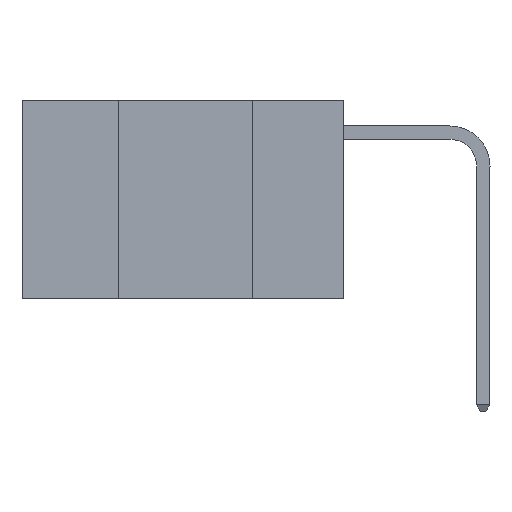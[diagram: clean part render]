
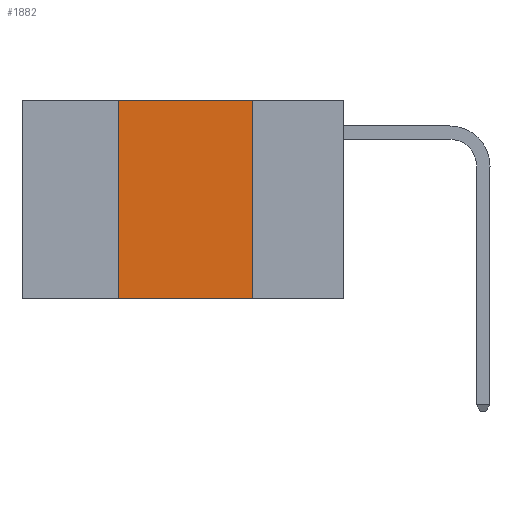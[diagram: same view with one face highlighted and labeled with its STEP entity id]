
A CAD part, left-side view. The second image highlights one B-rep face of the part: STEP entity #1882.
In plain terms, the highlighted planar face has unit normal (-1, 0, 0).
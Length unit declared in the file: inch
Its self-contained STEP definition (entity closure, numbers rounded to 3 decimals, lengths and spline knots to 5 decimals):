
#71 = EDGE_CURVE ( 'NONE', #2229, #2671, #3245, .T. ) ;
#581 = EDGE_CURVE ( 'NONE', #2229, #3153, #977, .T. ) ;
#640 = EDGE_LOOP ( 'NONE', ( #3433, #2370, #1067, #1055 ) ) ;
#672 = CARTESIAN_POINT ( 'NONE',  ( 0., 0.42, 0. ) ) ;
#694 = FACE_OUTER_BOUND ( 'NONE', #640, .T. ) ;
#722 = VECTOR ( 'NONE', #8742, 39.37008 ) ;
#977 = LINE ( 'NONE', #672, #722 ) ;
#986 = VECTOR ( 'NONE', #7277, 39.37008 ) ;
#1055 = ORIENTED_EDGE ( 'NONE', *, *, #71, .T. ) ;
#1067 = ORIENTED_EDGE ( 'NONE', *, *, #581, .F. ) ;
#1360 = AXIS2_PLACEMENT_3D ( 'NONE', #4078, #2463, #3861 ) ;
#1510 = CARTESIAN_POINT ( 'NONE',  ( 0., 0.42, 0. ) ) ;
#1602 = VERTEX_POINT ( 'NONE', #4942 ) ;
#1882 = ADVANCED_FACE ( 'NONE', ( #694 ), #4094, .F. ) ;
#2224 = DIRECTION ( 'NONE',  ( 0., 0., -1. ) ) ;
#2229 = VERTEX_POINT ( 'NONE', #7825 ) ;
#2370 = ORIENTED_EDGE ( 'NONE', *, *, #3351, .F. ) ;
#2463 = DIRECTION ( 'NONE',  ( 1., 0., 0. ) ) ;
#2671 = VERTEX_POINT ( 'NONE', #3814 ) ;
#3137 = EDGE_CURVE ( 'NONE', #1602, #2671, #6580, .T. ) ;
#3153 = VERTEX_POINT ( 'NONE', #1510 ) ;
#3245 = LINE ( 'NONE', #5629, #986 ) ;
#3351 = EDGE_CURVE ( 'NONE', #3153, #1602, #5281, .T. ) ;
#3433 = ORIENTED_EDGE ( 'NONE', *, *, #3137, .F. ) ;
#3814 = CARTESIAN_POINT ( 'NONE',  ( 0., 0.17, -0.37 ) ) ;
#3861 = DIRECTION ( 'NONE',  ( 0., 0., -1. ) ) ;
#4078 = CARTESIAN_POINT ( 'NONE',  ( 0., 0.6, 0. ) ) ;
#4094 = PLANE ( 'NONE',  #1360 ) ;
#4711 = CARTESIAN_POINT ( 'NONE',  ( 0., 0.6, 0. ) ) ;
#4942 = CARTESIAN_POINT ( 'NONE',  ( 0., 0.17, 0. ) ) ;
#5281 = LINE ( 'NONE', #4711, #8703 ) ;
#5454 = DIRECTION ( 'NONE',  ( 0., -1., 0. ) ) ;
#5629 = CARTESIAN_POINT ( 'NONE',  ( 0., 0.6, -0.37 ) ) ;
#6580 = LINE ( 'NONE', #7313, #8403 ) ;
#7277 = DIRECTION ( 'NONE',  ( 0., -1., 0. ) ) ;
#7313 = CARTESIAN_POINT ( 'NONE',  ( 0., 0.17, 0. ) ) ;
#7825 = CARTESIAN_POINT ( 'NONE',  ( 0., 0.42, -0.37 ) ) ;
#8403 = VECTOR ( 'NONE', #2224, 39.37008 ) ;
#8703 = VECTOR ( 'NONE', #5454, 39.37008 ) ;
#8742 = DIRECTION ( 'NONE',  ( 0., 0., 1. ) ) ;
